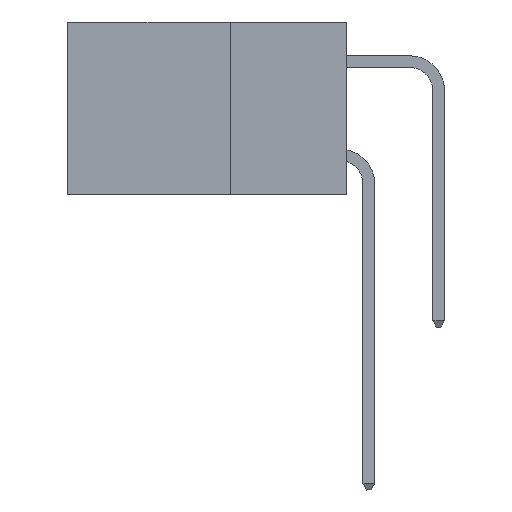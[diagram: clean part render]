
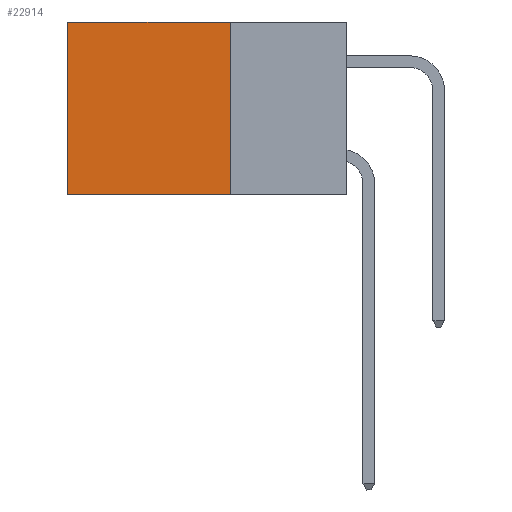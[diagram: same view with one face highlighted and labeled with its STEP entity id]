
A CAD part, left-side view. The second image highlights one B-rep face of the part: STEP entity #22914.
In plain terms, the highlighted planar face has unit normal (-1, 0, 0).
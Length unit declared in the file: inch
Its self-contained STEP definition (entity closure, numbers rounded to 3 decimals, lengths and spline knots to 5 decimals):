
#2222 = EDGE_CURVE ( 'NONE', #12634, #8749, #21817, .T. ) ;
#2663 = LINE ( 'NONE', #17181, #3251 ) ;
#3059 = CARTESIAN_POINT ( 'NONE',  ( 0.2875, 0.6, 0. ) ) ;
#3251 = VECTOR ( 'NONE', #19017, 39.37008 ) ;
#4589 = ORIENTED_EDGE ( 'NONE', *, *, #2222, .T. ) ;
#4735 = PLANE ( 'NONE',  #22644 ) ;
#4931 = DIRECTION ( 'NONE',  ( 0., 0., -1. ) ) ;
#5144 = CARTESIAN_POINT ( 'NONE',  ( 0.2875, 0.25, 0. ) ) ;
#5389 = EDGE_CURVE ( 'NONE', #20241, #23647, #12361, .T. ) ;
#5545 = DIRECTION ( 'NONE',  ( 0., 1., 0. ) ) ;
#6415 = DIRECTION ( 'NONE',  ( 0., 1., 0. ) ) ;
#7700 = CARTESIAN_POINT ( 'NONE',  ( 0.2875, 0.25, -0.37 ) ) ;
#8469 = DIRECTION ( 'NONE',  ( 0., 0., -1. ) ) ;
#8749 = VERTEX_POINT ( 'NONE', #12154 ) ;
#12154 = CARTESIAN_POINT ( 'NONE',  ( 0.2875, 0.6, 0. ) ) ;
#12361 = LINE ( 'NONE', #15024, #16174 ) ;
#12400 = FACE_OUTER_BOUND ( 'NONE', #16663, .T. ) ;
#12634 = VERTEX_POINT ( 'NONE', #5144 ) ;
#15024 = CARTESIAN_POINT ( 'NONE',  ( 0.2875, 0.25, -0.37 ) ) ;
#16174 = VECTOR ( 'NONE', #6415, 39.37008 ) ;
#16421 = EDGE_CURVE ( 'NONE', #12634, #20241, #2663, .T. ) ;
#16663 = EDGE_LOOP ( 'NONE', ( #19238, #23928, #20968, #4589 ) ) ;
#16741 = EDGE_CURVE ( 'NONE', #8749, #23647, #19929, .T. ) ;
#16894 = VECTOR ( 'NONE', #5545, 39.37008 ) ;
#17181 = CARTESIAN_POINT ( 'NONE',  ( 0.2875, 0.25, 0. ) ) ;
#17820 = CARTESIAN_POINT ( 'NONE',  ( 0.2875, 0.25, 0. ) ) ;
#19017 = DIRECTION ( 'NONE',  ( 0., 0., -1. ) ) ;
#19238 = ORIENTED_EDGE ( 'NONE', *, *, #16741, .T. ) ;
#19330 = VECTOR ( 'NONE', #4931, 39.37008 ) ;
#19643 = CARTESIAN_POINT ( 'NONE',  ( 0.2875, 0.25, 0. ) ) ;
#19727 = DIRECTION ( 'NONE',  ( 1., 0., 0. ) ) ;
#19929 = LINE ( 'NONE', #3059, #19330 ) ;
#20241 = VERTEX_POINT ( 'NONE', #7700 ) ;
#20968 = ORIENTED_EDGE ( 'NONE', *, *, #16421, .F. ) ;
#21817 = LINE ( 'NONE', #17820, #16894 ) ;
#22644 = AXIS2_PLACEMENT_3D ( 'NONE', #19643, #19727, #8469 ) ;
#22914 = ADVANCED_FACE ( 'NONE', ( #12400 ), #4735, .F. ) ;
#23647 = VERTEX_POINT ( 'NONE', #24060 ) ;
#23928 = ORIENTED_EDGE ( 'NONE', *, *, #5389, .F. ) ;
#24060 = CARTESIAN_POINT ( 'NONE',  ( 0.2875, 0.6, -0.37 ) ) ;
